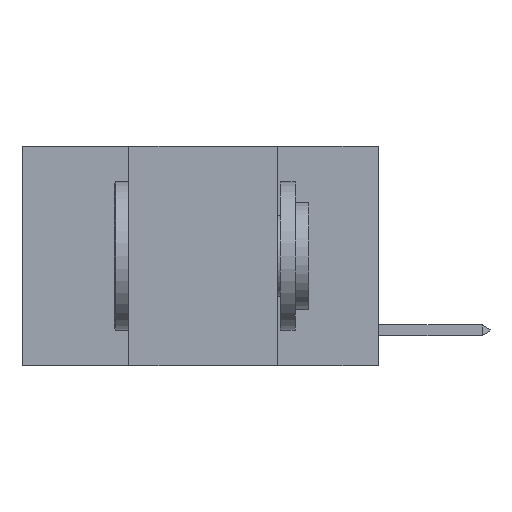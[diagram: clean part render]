
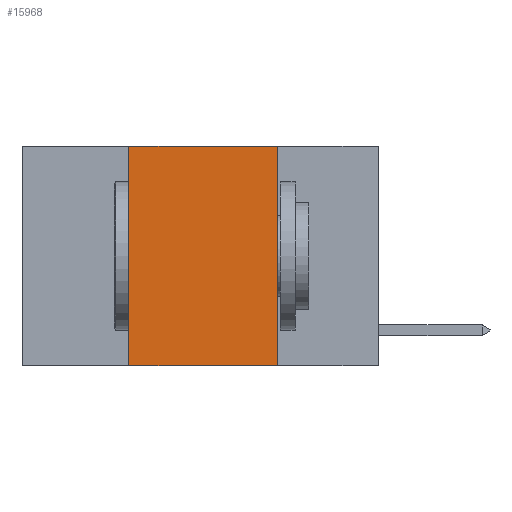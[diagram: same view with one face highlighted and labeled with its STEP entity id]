
A CAD part, left-side view. The second image highlights one B-rep face of the part: STEP entity #15968.
In plain terms, the highlighted planar face has unit normal (-1, 0, 0).
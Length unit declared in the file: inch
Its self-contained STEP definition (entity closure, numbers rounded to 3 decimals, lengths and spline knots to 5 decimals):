
#994 = VECTOR ( 'NONE', #17609, 39.37008 ) ;
#1753 = CARTESIAN_POINT ( 'NONE',  ( 0., 0.42, -0.37 ) ) ;
#3048 = VERTEX_POINT ( 'NONE', #21861 ) ;
#3120 = ORIENTED_EDGE ( 'NONE', *, *, #12974, .F. ) ;
#3400 = EDGE_CURVE ( 'NONE', #5042, #12457, #22779, .T. ) ;
#3712 = ORIENTED_EDGE ( 'NONE', *, *, #8657, .F. ) ;
#3883 = PLANE ( 'NONE',  #12286 ) ;
#4443 = CARTESIAN_POINT ( 'NONE',  ( 0., 0.6, 0. ) ) ;
#5042 = VERTEX_POINT ( 'NONE', #1753 ) ;
#5422 = FACE_OUTER_BOUND ( 'NONE', #14106, .T. ) ;
#5755 = ORIENTED_EDGE ( 'NONE', *, *, #3400, .T. ) ;
#6513 = DIRECTION ( 'NONE',  ( 1., 0., 0. ) ) ;
#8657 = EDGE_CURVE ( 'NONE', #3048, #23305, #12073, .T. ) ;
#9487 = LINE ( 'NONE', #15416, #994 ) ;
#10589 = DIRECTION ( 'NONE',  ( 0., 0., -1. ) ) ;
#10590 = VECTOR ( 'NONE', #10929, 39.37008 ) ;
#10929 = DIRECTION ( 'NONE',  ( 0., 0., 1. ) ) ;
#11422 = VECTOR ( 'NONE', #16598, 39.37008 ) ;
#12073 = LINE ( 'NONE', #27532, #11422 ) ;
#12286 = AXIS2_PLACEMENT_3D ( 'NONE', #4443, #6513, #10589 ) ;
#12457 = VERTEX_POINT ( 'NONE', #22122 ) ;
#12974 = EDGE_CURVE ( 'NONE', #23305, #12457, #9487, .T. ) ;
#13369 = DIRECTION ( 'NONE',  ( 0., -1., 0. ) ) ;
#14106 = EDGE_LOOP ( 'NONE', ( #3120, #3712, #20056, #5755 ) ) ;
#14442 = CARTESIAN_POINT ( 'NONE',  ( 0., 0.17, 0. ) ) ;
#15416 = CARTESIAN_POINT ( 'NONE',  ( 0., 0.17, 0. ) ) ;
#15968 = ADVANCED_FACE ( 'NONE', ( #5422 ), #3883, .F. ) ;
#16255 = LINE ( 'NONE', #23641, #10590 ) ;
#16598 = DIRECTION ( 'NONE',  ( 0., -1., 0. ) ) ;
#17609 = DIRECTION ( 'NONE',  ( 0., 0., -1. ) ) ;
#20056 = ORIENTED_EDGE ( 'NONE', *, *, #20682, .F. ) ;
#20682 = EDGE_CURVE ( 'NONE', #5042, #3048, #16255, .T. ) ;
#21861 = CARTESIAN_POINT ( 'NONE',  ( 0., 0.42, 0. ) ) ;
#22122 = CARTESIAN_POINT ( 'NONE',  ( 0., 0.17, -0.37 ) ) ;
#22779 = LINE ( 'NONE', #24358, #27170 ) ;
#23305 = VERTEX_POINT ( 'NONE', #14442 ) ;
#23641 = CARTESIAN_POINT ( 'NONE',  ( 0., 0.42, 0. ) ) ;
#24358 = CARTESIAN_POINT ( 'NONE',  ( 0., 0.6, -0.37 ) ) ;
#27170 = VECTOR ( 'NONE', #13369, 39.37008 ) ;
#27532 = CARTESIAN_POINT ( 'NONE',  ( 0., 0.6, 0. ) ) ;
